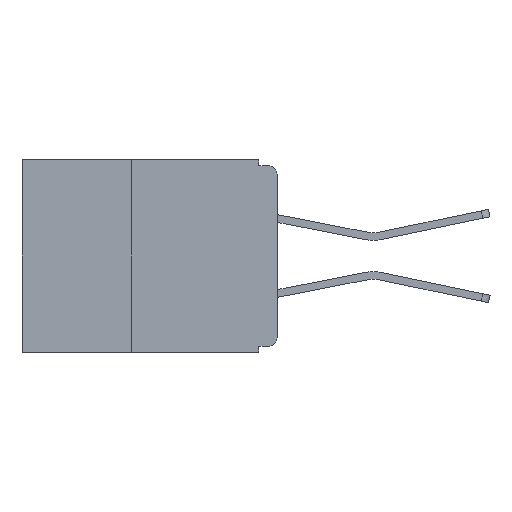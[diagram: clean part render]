
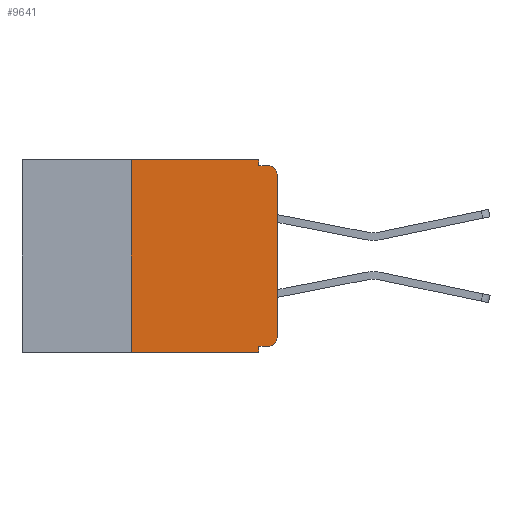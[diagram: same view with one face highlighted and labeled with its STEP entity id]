
A CAD part, left-side view. The second image highlights one B-rep face of the part: STEP entity #9641.
In plain terms, the highlighted planar face has unit normal (-1, 0, 0).
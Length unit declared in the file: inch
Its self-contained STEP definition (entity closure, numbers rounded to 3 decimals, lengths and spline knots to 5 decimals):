
#60 = ORIENTED_EDGE ( 'NONE', *, *, #8744, .T. ) ;
#122 = EDGE_CURVE ( 'NONE', #1312, #3344, #1076, .T. ) ;
#155 = CARTESIAN_POINT ( 'NONE',  ( 0., 0., -0.305 ) ) ;
#165 = CARTESIAN_POINT ( 'NONE',  ( 0., 0., -0.32 ) ) ;
#526 = LINE ( 'NONE', #6510, #6848 ) ;
#743 = DIRECTION ( 'NONE',  ( 0., 0., -1. ) ) ;
#1076 = CIRCLE ( 'NONE', #10411, 0.015 ) ;
#1183 = ORIENTED_EDGE ( 'NONE', *, *, #5893, .F. ) ;
#1312 = VERTEX_POINT ( 'NONE', #4570 ) ;
#1381 = ORIENTED_EDGE ( 'NONE', *, *, #122, .T. ) ;
#1450 = VERTEX_POINT ( 'NONE', #3123 ) ;
#1888 = AXIS2_PLACEMENT_3D ( 'NONE', #7418, #2292, #3127 ) ;
#1925 = EDGE_CURVE ( 'NONE', #1312, #3915, #7824, .T. ) ;
#2292 = DIRECTION ( 'NONE',  ( 1., 0., 0. ) ) ;
#2316 = ORIENTED_EDGE ( 'NONE', *, *, #10906, .F. ) ;
#2322 = CARTESIAN_POINT ( 'NONE',  ( 0., 0.031, -0.32 ) ) ;
#2490 = FACE_OUTER_BOUND ( 'NONE', #9951, .T. ) ;
#2614 = DIRECTION ( 'NONE',  ( 0., -1., 0. ) ) ;
#2711 = CARTESIAN_POINT ( 'NONE',  ( 0., 0.015, -0.025 ) ) ;
#2979 = VECTOR ( 'NONE', #9542, 39.37008 ) ;
#3052 = PLANE ( 'NONE',  #1888 ) ;
#3123 = CARTESIAN_POINT ( 'NONE',  ( 0., 0.015, -0.01 ) ) ;
#3127 = DIRECTION ( 'NONE',  ( 0., 0., -1. ) ) ;
#3156 = VECTOR ( 'NONE', #8582, 39.37008 ) ;
#3249 = DIRECTION ( 'NONE',  ( 0., 0., 1. ) ) ;
#3303 = VERTEX_POINT ( 'NONE', #3648 ) ;
#3344 = VERTEX_POINT ( 'NONE', #155 ) ;
#3440 = VERTEX_POINT ( 'NONE', #10643 ) ;
#3489 = CARTESIAN_POINT ( 'NONE',  ( 0., 0., -0.025 ) ) ;
#3601 = VECTOR ( 'NONE', #8884, 39.37008 ) ;
#3648 = CARTESIAN_POINT ( 'NONE',  ( 0., 0.031, 0. ) ) ;
#3915 = VERTEX_POINT ( 'NONE', #2322 ) ;
#4310 = CARTESIAN_POINT ( 'NONE',  ( 0., 0.031, -0.01 ) ) ;
#4398 = CARTESIAN_POINT ( 'NONE',  ( 0., 0.437, -0.33 ) ) ;
#4438 = AXIS2_PLACEMENT_3D ( 'NONE', #2711, #10335, #9574 ) ;
#4570 = CARTESIAN_POINT ( 'NONE',  ( 0., 0.015, -0.32 ) ) ;
#4828 = DIRECTION ( 'NONE',  ( 0., -1., 0. ) ) ;
#4922 = VERTEX_POINT ( 'NONE', #9374 ) ;
#4989 = CARTESIAN_POINT ( 'NONE',  ( 0., 0.031, 0. ) ) ;
#5207 = ORIENTED_EDGE ( 'NONE', *, *, #10884, .T. ) ;
#5545 = VERTEX_POINT ( 'NONE', #3489 ) ;
#5813 = CARTESIAN_POINT ( 'NONE',  ( 0., 0.031, -0.33 ) ) ;
#5881 = CARTESIAN_POINT ( 'NONE',  ( 0., 0.015, -0.305 ) ) ;
#5893 = EDGE_CURVE ( 'NONE', #3440, #4922, #9013, .T. ) ;
#5908 = VECTOR ( 'NONE', #10169, 39.37008 ) ;
#5958 = EDGE_CURVE ( 'NONE', #3440, #9873, #6852, .T. ) ;
#6510 = CARTESIAN_POINT ( 'NONE',  ( 0., 0.437, 0. ) ) ;
#6793 = VERTEX_POINT ( 'NONE', #4310 ) ;
#6807 = LINE ( 'NONE', #4989, #3156 ) ;
#6848 = VECTOR ( 'NONE', #4828, 39.37008 ) ;
#6852 = LINE ( 'NONE', #4398, #7519 ) ;
#7140 = CARTESIAN_POINT ( 'NONE',  ( 0., 0., 0. ) ) ;
#7174 = EDGE_CURVE ( 'NONE', #3915, #9873, #8174, .T. ) ;
#7418 = CARTESIAN_POINT ( 'NONE',  ( 0., 0.437, 0. ) ) ;
#7472 = CIRCLE ( 'NONE', #4438, 0.015 ) ;
#7519 = VECTOR ( 'NONE', #2614, 39.37008 ) ;
#7824 = LINE ( 'NONE', #165, #2979 ) ;
#7962 = DIRECTION ( 'NONE',  ( 0., -1., 0. ) ) ;
#8001 = CARTESIAN_POINT ( 'NONE',  ( 0., 0., -0.01 ) ) ;
#8174 = LINE ( 'NONE', #5813, #5908 ) ;
#8577 = EDGE_CURVE ( 'NONE', #3303, #6793, #6807, .T. ) ;
#8582 = DIRECTION ( 'NONE',  ( 0., 0., -1. ) ) ;
#8676 = CARTESIAN_POINT ( 'NONE',  ( 0., 0.031, -0.33 ) ) ;
#8714 = VECTOR ( 'NONE', #7962, 39.37008 ) ;
#8744 = EDGE_CURVE ( 'NONE', #5545, #1450, #7472, .T. ) ;
#8804 = ORIENTED_EDGE ( 'NONE', *, *, #1925, .F. ) ;
#8873 = ORIENTED_EDGE ( 'NONE', *, *, #8577, .F. ) ;
#8884 = DIRECTION ( 'NONE',  ( 0., 0., 1. ) ) ;
#9013 = LINE ( 'NONE', #10208, #10996 ) ;
#9374 = CARTESIAN_POINT ( 'NONE',  ( 0., 0.25, 0. ) ) ;
#9542 = DIRECTION ( 'NONE',  ( 0., 1., 0. ) ) ;
#9574 = DIRECTION ( 'NONE',  ( 0., 0., -1. ) ) ;
#9641 = ADVANCED_FACE ( 'NONE', ( #2490 ), #3052, .F. ) ;
#9873 = VERTEX_POINT ( 'NONE', #8676 ) ;
#9951 = EDGE_LOOP ( 'NONE', ( #5207, #60, #2316, #8873, #9964, #1183, #10158, #10170, #8804, #1381 ) ) ;
#9964 = ORIENTED_EDGE ( 'NONE', *, *, #10565, .F. ) ;
#10158 = ORIENTED_EDGE ( 'NONE', *, *, #5958, .T. ) ;
#10169 = DIRECTION ( 'NONE',  ( 0., 0., -1. ) ) ;
#10170 = ORIENTED_EDGE ( 'NONE', *, *, #7174, .F. ) ;
#10208 = CARTESIAN_POINT ( 'NONE',  ( 0., 0.25, -0.33 ) ) ;
#10329 = LINE ( 'NONE', #7140, #3601 ) ;
#10335 = DIRECTION ( 'NONE',  ( -1., 0., 0. ) ) ;
#10411 = AXIS2_PLACEMENT_3D ( 'NONE', #5881, #11113, #743 ) ;
#10565 = EDGE_CURVE ( 'NONE', #4922, #3303, #526, .T. ) ;
#10643 = CARTESIAN_POINT ( 'NONE',  ( 0., 0.25, -0.33 ) ) ;
#10884 = EDGE_CURVE ( 'NONE', #3344, #5545, #10329, .T. ) ;
#10906 = EDGE_CURVE ( 'NONE', #6793, #1450, #10981, .T. ) ;
#10981 = LINE ( 'NONE', #8001, #8714 ) ;
#10996 = VECTOR ( 'NONE', #3249, 39.37008 ) ;
#11113 = DIRECTION ( 'NONE',  ( -1., 0., 0. ) ) ;
